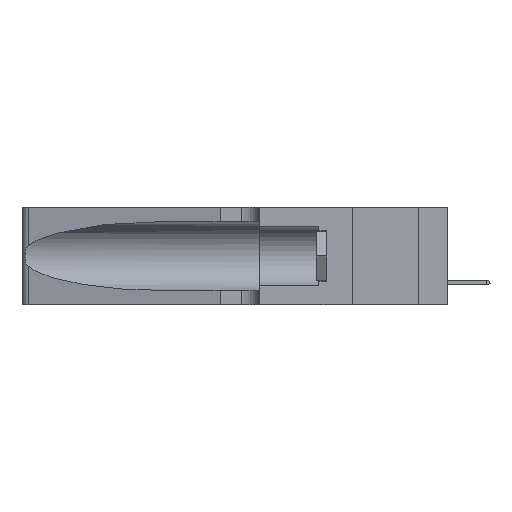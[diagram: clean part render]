
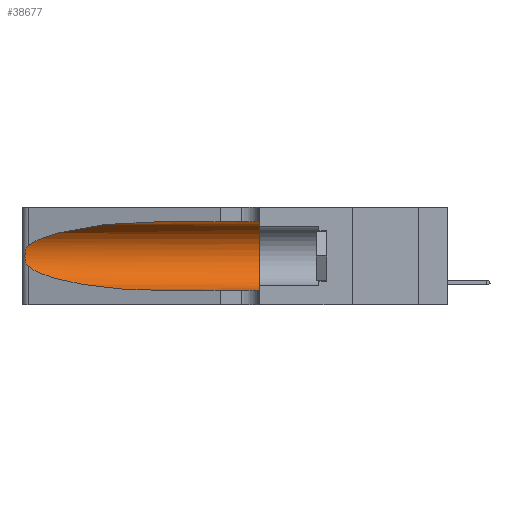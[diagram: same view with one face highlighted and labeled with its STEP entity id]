
A CAD part, left-side view. The second image highlights one B-rep face of the part: STEP entity #38677.
In plain terms, the highlighted cylindrical face has radius 3.308 mm (diameter 6.617 mm), a partial arc.
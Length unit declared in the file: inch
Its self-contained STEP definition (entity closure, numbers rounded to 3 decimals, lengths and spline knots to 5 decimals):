
#21 = VERTEX_POINT ( 'NONE', #30016 ) ;
#224 = DIRECTION ( 'NONE',  ( 0., 0., -1. ) ) ;
#811 = CARTESIAN_POINT ( 'NONE',  ( 0.1305, 0.72297, 0.31525 ) ) ;
#1100 = CARTESIAN_POINT ( 'NONE',  ( 0.1305, 0.72297, 0.05475 ) ) ;
#2966 = CARTESIAN_POINT ( 'NONE',  ( 0.25789, 1.23486, 0.15765 ) ) ;
#5582 =( BOUNDED_CURVE ( )  B_SPLINE_CURVE ( 3, ( #811, #33439, #40398, #28441 ),
 .UNSPECIFIED., .F., .F. ) 
 B_SPLINE_CURVE_WITH_KNOTS ( ( 4, 4 ),
 ( 1.5708, 2.84003 ),
 .UNSPECIFIED. ) 
 CURVE ( )  GEOMETRIC_REPRESENTATION_ITEM ( )  RATIONAL_B_SPLINE_CURVE ( ( 1., 0.87, 0.87, 1. ) ) 
 REPRESENTATION_ITEM ( '' )  );
#5760 = VERTEX_POINT ( 'NONE', #9362 ) ;
#6235 = CARTESIAN_POINT ( 'NONE',  ( 0.26018, 1.23835, 0.19895 ) ) ;
#6303 = CARTESIAN_POINT ( 'NONE',  ( 0.1305, 0.35, 0.185 ) ) ;
#6785 = AXIS2_PLACEMENT_3D ( 'NONE', #33015, #19153, #224 ) ;
#7290 = CIRCLE ( 'NONE', #26526, 0.13025 ) ;
#7887 = ORIENTED_EDGE ( 'NONE', *, *, #25085, .T. ) ;
#8492 = ORIENTED_EDGE ( 'NONE', *, *, #10622, .F. ) ;
#8703 = CARTESIAN_POINT ( 'NONE',  ( 0.1305, 0.72297, 0.05475 ) ) ;
#9362 = CARTESIAN_POINT ( 'NONE',  ( 0.1305, 0.35, 0.05475 ) ) ;
#9561 = CARTESIAN_POINT ( 'NONE',  ( 0.26017, 1.23833, 0.17102 ) ) ;
#10167 = CARTESIAN_POINT ( 'NONE',  ( 0.25487, 1.22718, 0.22369 ) ) ;
#10599 = CARTESIAN_POINT ( 'NONE',  ( 0.25639, 1.23184, 0.21858 ) ) ;
#10622 = EDGE_CURVE ( 'NONE', #37081, #5760, #7290, .T. ) ;
#13132 = VERTEX_POINT ( 'NONE', #24843 ) ;
#13154 = DIRECTION ( 'NONE',  ( 0., -1., 0. ) ) ;
#13739 = ORIENTED_EDGE ( 'NONE', *, *, #37414, .F. ) ;
#15525 = VECTOR ( 'NONE', #28070, 39.37008 ) ;
#15861 = CARTESIAN_POINT ( 'NONE',  ( 0.25787, 1.23484, 0.2124 ) ) ;
#16403 = CARTESIAN_POINT ( 'NONE',  ( 0.25639, 1.23186, 0.15144 ) ) ;
#18144 = VECTOR ( 'NONE', #13154, 39.37008 ) ;
#18256 = VERTEX_POINT ( 'NONE', #8703 ) ;
#18428 = ORIENTED_EDGE ( 'NONE', *, *, #34938, .T. ) ;
#19153 = DIRECTION ( 'NONE',  ( 0., -1., 0. ) ) ;
#19945 = CARTESIAN_POINT ( 'NONE',  ( 0.26075, 1.23896, 0.178 ) ) ;
#20835 = CARTESIAN_POINT ( 'NONE',  ( 0.25555, 1.22994, 0.2215 ) ) ;
#20940 = EDGE_CURVE ( 'NONE', #13132, #18256, #29164, .T. ) ;
#22729 = CARTESIAN_POINT ( 'NONE',  ( 0.25555, 1.22993, 0.14849 ) ) ;
#24843 = CARTESIAN_POINT ( 'NONE',  ( 0.25487, 1.22718, 0.14631 ) ) ;
#24926 = LINE ( 'NONE', #25668, #15525 ) ;
#25085 = EDGE_CURVE ( 'NONE', #18256, #5760, #24926, .T. ) ;
#25122 = CARTESIAN_POINT ( 'NONE',  ( 0.18966, 0.96281, 0.05475 ) ) ;
#25668 = CARTESIAN_POINT ( 'NONE',  ( 0.1305, 1.61858, 0.05475 ) ) ;
#26084 = CARTESIAN_POINT ( 'NONE',  ( 0.26075, 1.23896, 0.19203 ) ) ;
#26508 = CARTESIAN_POINT ( 'NONE',  ( 0.25854, 1.2359, 0.20912 ) ) ;
#26526 = AXIS2_PLACEMENT_3D ( 'NONE', #6303, #36478, #31493 ) ;
#28070 = DIRECTION ( 'NONE',  ( 0., -1., 0. ) ) ;
#28395 = CARTESIAN_POINT ( 'NONE',  ( 0.1305, 0.35, 0.31525 ) ) ;
#28441 = CARTESIAN_POINT ( 'NONE',  ( 0.25487, 1.22718, 0.22369 ) ) ;
#28739 = ORIENTED_EDGE ( 'NONE', *, *, #20940, .T. ) ;
#29164 =( BOUNDED_CURVE ( )  B_SPLINE_CURVE ( 3, ( #41590, #34997, #25122, #1100 ),
 .UNSPECIFIED., .F., .F. ) 
 B_SPLINE_CURVE_WITH_KNOTS ( ( 4, 4 ),
 ( 3.44316, 4.71239 ),
 .UNSPECIFIED. ) 
 CURVE ( )  GEOMETRIC_REPRESENTATION_ITEM ( )  RATIONAL_B_SPLINE_CURVE ( ( 1., 0.87, 0.87, 1. ) ) 
 REPRESENTATION_ITEM ( '' )  );
#29405 = B_SPLINE_CURVE_WITH_KNOTS ( 'NONE', 3,
 ( #10167, #20835, #10599, #15861, #26508, #6235, #26084, #19945, #9561, #32625, #2966, #16403, #22729, #33062 ),
 .UNSPECIFIED., .F., .F.,
 ( 4, 2, 2, 2, 2, 2, 4 ),
 ( 0., 0.00027, 0.00053, 0.00107, 0.0016, 0.00187, 0.00214 ),
 .UNSPECIFIED. ) ;
#30016 = CARTESIAN_POINT ( 'NONE',  ( 0.25487, 1.22718, 0.22369 ) ) ;
#30423 = EDGE_CURVE ( 'NONE', #40258, #21, #5582, .T. ) ;
#31493 = DIRECTION ( 'NONE',  ( 0., 0., 1. ) ) ;
#32625 = CARTESIAN_POINT ( 'NONE',  ( 0.25856, 1.23593, 0.16098 ) ) ;
#33015 = CARTESIAN_POINT ( 'NONE',  ( 0.1305, 1.61858, 0.185 ) ) ;
#33062 = CARTESIAN_POINT ( 'NONE',  ( 0.25487, 1.22718, 0.14631 ) ) ;
#33439 = CARTESIAN_POINT ( 'NONE',  ( 0.18966, 0.96281, 0.31525 ) ) ;
#34938 = EDGE_CURVE ( 'NONE', #21, #13132, #29405, .T. ) ;
#34997 = CARTESIAN_POINT ( 'NONE',  ( 0.2373, 1.15595, 0.08982 ) ) ;
#35333 = FACE_OUTER_BOUND ( 'NONE', #42228, .T. ) ;
#35781 = CARTESIAN_POINT ( 'NONE',  ( 0.1305, 1.61858, 0.31525 ) ) ;
#36478 = DIRECTION ( 'NONE',  ( 0., 1., 0. ) ) ;
#37081 = VERTEX_POINT ( 'NONE', #28395 ) ;
#37414 = EDGE_CURVE ( 'NONE', #40258, #37081, #37979, .T. ) ;
#37979 = LINE ( 'NONE', #35781, #18144 ) ;
#38677 = ADVANCED_FACE ( 'NONE', ( #35333 ), #42690, .F. ) ;
#39784 = ORIENTED_EDGE ( 'NONE', *, *, #30423, .T. ) ;
#40258 = VERTEX_POINT ( 'NONE', #41960 ) ;
#40398 = CARTESIAN_POINT ( 'NONE',  ( 0.2373, 1.15595, 0.28018 ) ) ;
#41590 = CARTESIAN_POINT ( 'NONE',  ( 0.25487, 1.22718, 0.14631 ) ) ;
#41960 = CARTESIAN_POINT ( 'NONE',  ( 0.1305, 0.72297, 0.31525 ) ) ;
#42228 = EDGE_LOOP ( 'NONE', ( #39784, #18428, #28739, #7887, #8492, #13739 ) ) ;
#42690 = CYLINDRICAL_SURFACE ( 'NONE', #6785, 0.13025 ) ;
